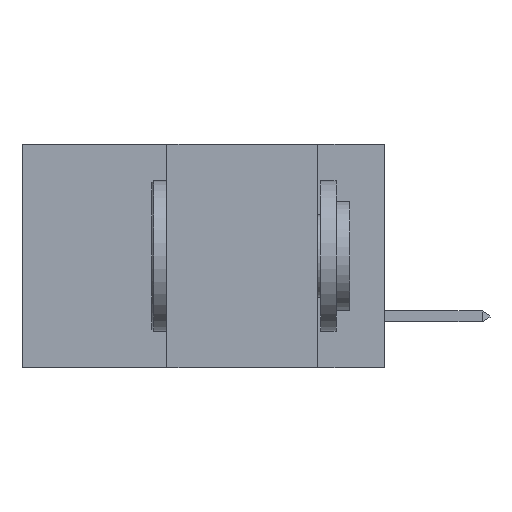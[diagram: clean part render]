
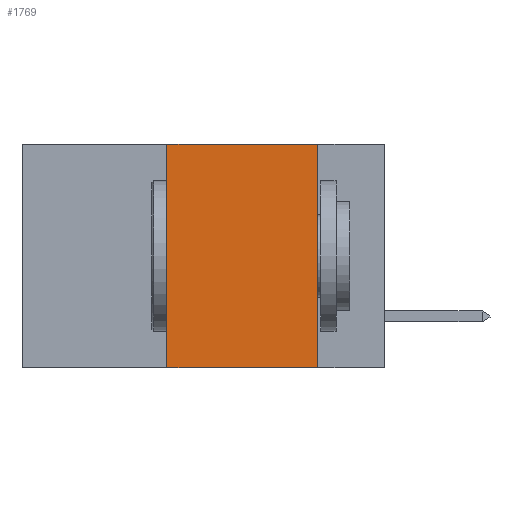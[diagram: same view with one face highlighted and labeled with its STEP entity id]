
A CAD part, left-side view. The second image highlights one B-rep face of the part: STEP entity #1769.
In plain terms, the highlighted planar face has unit normal (-1, 0, 0).
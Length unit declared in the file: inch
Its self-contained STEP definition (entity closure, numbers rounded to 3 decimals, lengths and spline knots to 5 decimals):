
#33 = VERTEX_POINT ( 'NONE', #1037 ) ;
#493 = CARTESIAN_POINT ( 'NONE',  ( 0., 0.36, 0. ) ) ;
#1037 = CARTESIAN_POINT ( 'NONE',  ( 0., 0.11, 0. ) ) ;
#1598 = CARTESIAN_POINT ( 'NONE',  ( 0., 0.36, 0. ) ) ;
#1769 = ADVANCED_FACE ( 'NONE', ( #10275 ), #7348, .F. ) ;
#1946 = DIRECTION ( 'NONE',  ( 0., -1., 0. ) ) ;
#2350 = DIRECTION ( 'NONE',  ( 0., 0., -1. ) ) ;
#2548 = VECTOR ( 'NONE', #1946, 39.37008 ) ;
#2664 = VERTEX_POINT ( 'NONE', #493 ) ;
#2696 = ORIENTED_EDGE ( 'NONE', *, *, #10227, .F. ) ;
#2767 = ORIENTED_EDGE ( 'NONE', *, *, #7208, .F. ) ;
#2790 = ORIENTED_EDGE ( 'NONE', *, *, #9751, .F. ) ;
#2824 = ORIENTED_EDGE ( 'NONE', *, *, #6786, .T. ) ;
#2901 = VECTOR ( 'NONE', #8135, 39.37008 ) ;
#3077 = CARTESIAN_POINT ( 'NONE',  ( 0., 0.36, -0.37 ) ) ;
#3440 = AXIS2_PLACEMENT_3D ( 'NONE', #8200, #6249, #6127 ) ;
#4716 = LINE ( 'NONE', #7677, #2548 ) ;
#4767 = CARTESIAN_POINT ( 'NONE',  ( 0., 0.6, 0. ) ) ;
#5467 = LINE ( 'NONE', #7277, #9558 ) ;
#5712 = EDGE_LOOP ( 'NONE', ( #2696, #2767, #2790, #2824 ) ) ;
#6127 = DIRECTION ( 'NONE',  ( 0., 0., -1. ) ) ;
#6249 = DIRECTION ( 'NONE',  ( 1., 0., 0. ) ) ;
#6475 = DIRECTION ( 'NONE',  ( 0., -1., 0. ) ) ;
#6786 = EDGE_CURVE ( 'NONE', #8915, #9999, #4716, .T. ) ;
#6939 = VECTOR ( 'NONE', #6475, 39.37008 ) ;
#7208 = EDGE_CURVE ( 'NONE', #2664, #33, #8927, .T. ) ;
#7277 = CARTESIAN_POINT ( 'NONE',  ( 0., 0.11, 0. ) ) ;
#7348 = PLANE ( 'NONE',  #3440 ) ;
#7677 = CARTESIAN_POINT ( 'NONE',  ( 0., 0.6, -0.37 ) ) ;
#8135 = DIRECTION ( 'NONE',  ( 0., 0., 1. ) ) ;
#8200 = CARTESIAN_POINT ( 'NONE',  ( 0., 0.6, 0. ) ) ;
#8915 = VERTEX_POINT ( 'NONE', #3077 ) ;
#8927 = LINE ( 'NONE', #4767, #6939 ) ;
#9218 = CARTESIAN_POINT ( 'NONE',  ( 0., 0.11, -0.37 ) ) ;
#9459 = LINE ( 'NONE', #1598, #2901 ) ;
#9558 = VECTOR ( 'NONE', #2350, 39.37008 ) ;
#9751 = EDGE_CURVE ( 'NONE', #8915, #2664, #9459, .T. ) ;
#9999 = VERTEX_POINT ( 'NONE', #9218 ) ;
#10227 = EDGE_CURVE ( 'NONE', #33, #9999, #5467, .T. ) ;
#10275 = FACE_OUTER_BOUND ( 'NONE', #5712, .T. ) ;
